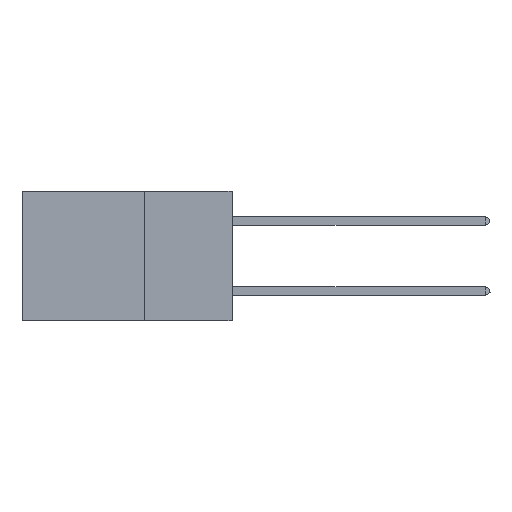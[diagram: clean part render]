
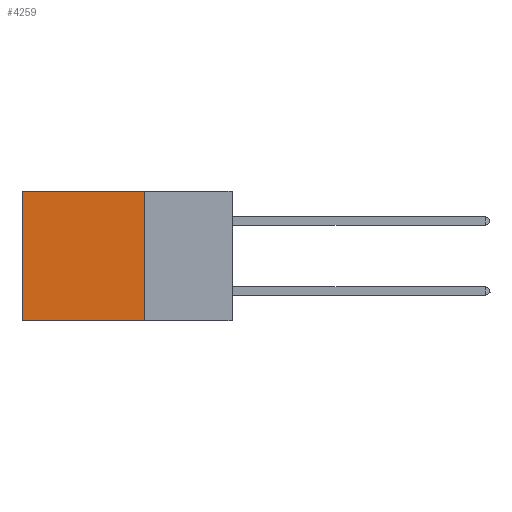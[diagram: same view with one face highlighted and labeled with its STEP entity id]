
A CAD part, left-side view. The second image highlights one B-rep face of the part: STEP entity #4259.
In plain terms, the highlighted planar face has unit normal (-1, 0, 0).
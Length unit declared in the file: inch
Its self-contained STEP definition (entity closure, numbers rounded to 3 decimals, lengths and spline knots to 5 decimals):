
#610 = CARTESIAN_POINT ( 'NONE',  ( 0.2875, 0.25, 0. ) ) ;
#1632 = EDGE_CURVE ( 'NONE', #4852, #7119, #17567, .T. ) ;
#1838 = DIRECTION ( 'NONE',  ( 1., 0., 0. ) ) ;
#1875 = VECTOR ( 'NONE', #15494, 39.37008 ) ;
#2458 = VECTOR ( 'NONE', #26870, 39.37008 ) ;
#2823 = EDGE_CURVE ( 'NONE', #16075, #5789, #22762, .T. ) ;
#4259 = ADVANCED_FACE ( 'NONE', ( #4963 ), #28137, .F. ) ;
#4852 = VERTEX_POINT ( 'NONE', #9825 ) ;
#4963 = FACE_OUTER_BOUND ( 'NONE', #25184, .T. ) ;
#4974 = EDGE_CURVE ( 'NONE', #4852, #16075, #21513, .T. ) ;
#5210 = CARTESIAN_POINT ( 'NONE',  ( 0.2875, 0.25, -0.37 ) ) ;
#5789 = VERTEX_POINT ( 'NONE', #25059 ) ;
#6534 = ORIENTED_EDGE ( 'NONE', *, *, #2823, .F. ) ;
#6872 = VECTOR ( 'NONE', #18501, 39.37008 ) ;
#7119 = VERTEX_POINT ( 'NONE', #8220 ) ;
#7457 = VECTOR ( 'NONE', #16444, 39.37008 ) ;
#8108 = ORIENTED_EDGE ( 'NONE', *, *, #4974, .F. ) ;
#8220 = CARTESIAN_POINT ( 'NONE',  ( 0.2875, 0.6, 0. ) ) ;
#8801 = CARTESIAN_POINT ( 'NONE',  ( 0.2875, 0.25, -0.37 ) ) ;
#9825 = CARTESIAN_POINT ( 'NONE',  ( 0.2875, 0.25, 0. ) ) ;
#10303 = EDGE_CURVE ( 'NONE', #7119, #5789, #22963, .T. ) ;
#10608 = AXIS2_PLACEMENT_3D ( 'NONE', #10925, #1838, #19350 ) ;
#10925 = CARTESIAN_POINT ( 'NONE',  ( 0.2875, 0.25, 0. ) ) ;
#14302 = CARTESIAN_POINT ( 'NONE',  ( 0.2875, 0.6, 0. ) ) ;
#15494 = DIRECTION ( 'NONE',  ( 0., 1., 0. ) ) ;
#16075 = VERTEX_POINT ( 'NONE', #5210 ) ;
#16444 = DIRECTION ( 'NONE',  ( 0., 0., -1. ) ) ;
#17567 = LINE ( 'NONE', #22884, #2458 ) ;
#18501 = DIRECTION ( 'NONE',  ( 0., 0., -1. ) ) ;
#19350 = DIRECTION ( 'NONE',  ( 0., 0., -1. ) ) ;
#21513 = LINE ( 'NONE', #610, #7457 ) ;
#22762 = LINE ( 'NONE', #8801, #1875 ) ;
#22884 = CARTESIAN_POINT ( 'NONE',  ( 0.2875, 0.25, 0. ) ) ;
#22963 = LINE ( 'NONE', #14302, #6872 ) ;
#25059 = CARTESIAN_POINT ( 'NONE',  ( 0.2875, 0.6, -0.37 ) ) ;
#25184 = EDGE_LOOP ( 'NONE', ( #26258, #6534, #8108, #25570 ) ) ;
#25570 = ORIENTED_EDGE ( 'NONE', *, *, #1632, .T. ) ;
#26258 = ORIENTED_EDGE ( 'NONE', *, *, #10303, .T. ) ;
#26870 = DIRECTION ( 'NONE',  ( 0., 1., 0. ) ) ;
#28137 = PLANE ( 'NONE',  #10608 ) ;
